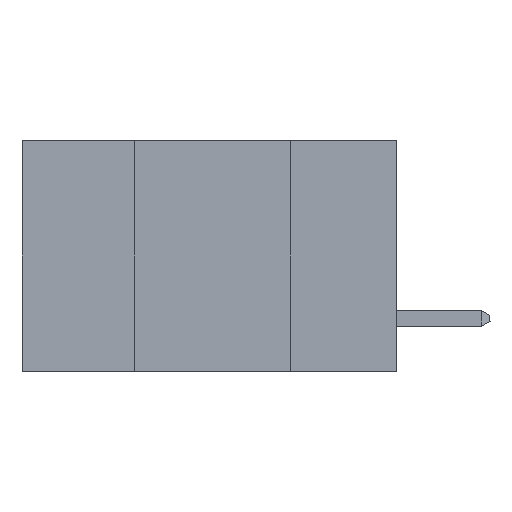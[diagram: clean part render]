
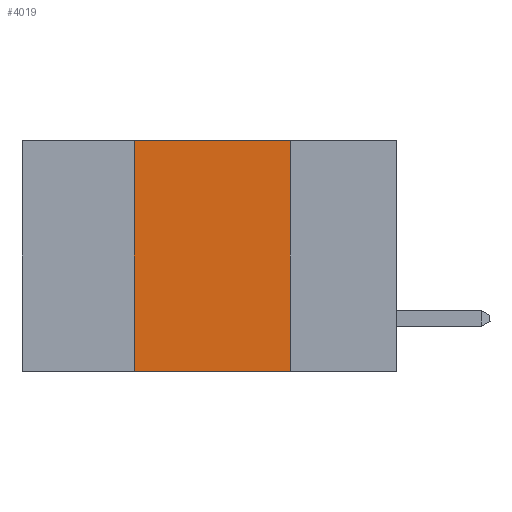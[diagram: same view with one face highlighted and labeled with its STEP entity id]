
A CAD part, left-side view. The second image highlights one B-rep face of the part: STEP entity #4019.
In plain terms, the highlighted planar face has unit normal (-1, 0, 0).
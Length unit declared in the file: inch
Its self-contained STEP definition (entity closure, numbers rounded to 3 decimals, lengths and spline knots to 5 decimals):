
#1301 = VERTEX_POINT ( 'NONE', #10527 ) ;
#1570 = EDGE_CURVE ( 'NONE', #10856, #11387, #16027, .T. ) ;
#2547 = LINE ( 'NONE', #14661, #6498 ) ;
#3858 = VERTEX_POINT ( 'NONE', #13329 ) ;
#4019 = ADVANCED_FACE ( 'NONE', ( #4283 ), #9472, .F. ) ;
#4283 = FACE_OUTER_BOUND ( 'NONE', #15941, .T. ) ;
#6093 = ORIENTED_EDGE ( 'NONE', *, *, #1570, .F. ) ;
#6498 = VECTOR ( 'NONE', #14561, 39.37008 ) ;
#6548 = ORIENTED_EDGE ( 'NONE', *, *, #15410, .T. ) ;
#8179 = CARTESIAN_POINT ( 'NONE',  ( 0., 0.42, 0. ) ) ;
#8919 = ORIENTED_EDGE ( 'NONE', *, *, #9336, .F. ) ;
#9336 = EDGE_CURVE ( 'NONE', #1301, #3858, #2547, .T. ) ;
#9472 = PLANE ( 'NONE',  #18127 ) ;
#9555 = VECTOR ( 'NONE', #12682, 39.37008 ) ;
#9957 = VECTOR ( 'NONE', #18093, 39.37008 ) ;
#10497 = DIRECTION ( 'NONE',  ( 0., 0., 1. ) ) ;
#10527 = CARTESIAN_POINT ( 'NONE',  ( 0., 0.17, 0. ) ) ;
#10856 = VERTEX_POINT ( 'NONE', #12189 ) ;
#11235 = CARTESIAN_POINT ( 'NONE',  ( 0., 0.6, -0.37 ) ) ;
#11387 = VERTEX_POINT ( 'NONE', #8179 ) ;
#12189 = CARTESIAN_POINT ( 'NONE',  ( 0., 0.42, -0.37 ) ) ;
#12404 = VECTOR ( 'NONE', #10497, 39.37008 ) ;
#12619 = CARTESIAN_POINT ( 'NONE',  ( 0., 0.6, 0. ) ) ;
#12682 = DIRECTION ( 'NONE',  ( 0., -1., 0. ) ) ;
#12765 = CARTESIAN_POINT ( 'NONE',  ( 0., 0.42, 0. ) ) ;
#12790 = CARTESIAN_POINT ( 'NONE',  ( 0., 0.6, 0. ) ) ;
#13329 = CARTESIAN_POINT ( 'NONE',  ( 0., 0.17, -0.37 ) ) ;
#13816 = LINE ( 'NONE', #12619, #9957 ) ;
#13863 = LINE ( 'NONE', #11235, #9555 ) ;
#14561 = DIRECTION ( 'NONE',  ( 0., 0., -1. ) ) ;
#14661 = CARTESIAN_POINT ( 'NONE',  ( 0., 0.17, 0. ) ) ;
#15410 = EDGE_CURVE ( 'NONE', #10856, #3858, #13863, .T. ) ;
#15941 = EDGE_LOOP ( 'NONE', ( #8919, #16428, #6093, #6548 ) ) ;
#16027 = LINE ( 'NONE', #12765, #12404 ) ;
#16428 = ORIENTED_EDGE ( 'NONE', *, *, #17184, .F. ) ;
#17081 = DIRECTION ( 'NONE',  ( 0., 0., -1. ) ) ;
#17184 = EDGE_CURVE ( 'NONE', #11387, #1301, #13816, .T. ) ;
#17244 = DIRECTION ( 'NONE',  ( 1., 0., 0. ) ) ;
#18093 = DIRECTION ( 'NONE',  ( 0., -1., 0. ) ) ;
#18127 = AXIS2_PLACEMENT_3D ( 'NONE', #12790, #17244, #17081 ) ;
